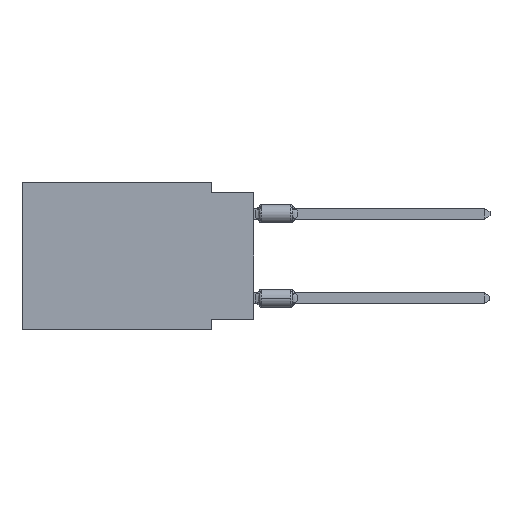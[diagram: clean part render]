
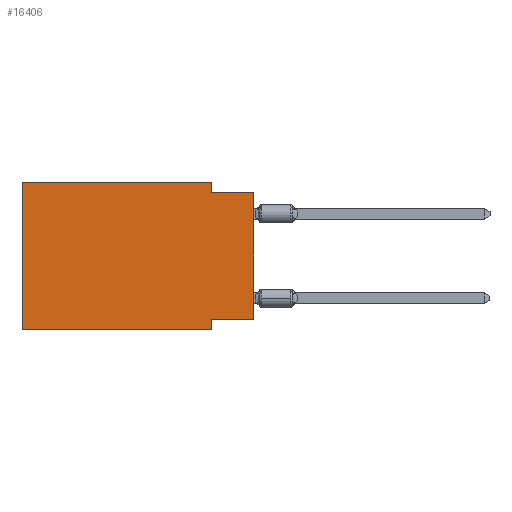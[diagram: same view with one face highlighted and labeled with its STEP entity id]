
A CAD part, left-side view. The second image highlights one B-rep face of the part: STEP entity #16406.
In plain terms, the highlighted planar face has unit normal (-1, 0, 0).
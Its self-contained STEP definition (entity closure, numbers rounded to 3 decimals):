
#138 = VERTEX_POINT ( 'NONE', #2093 ) ;
#1207 = EDGE_CURVE ( 'NONE', #15112, #24728, #23147, .T. ) ;
#1878 = VECTOR ( 'NONE', #22965, 1000. ) ;
#2093 = CARTESIAN_POINT ( 'NONE',  ( 0., 2.54, -0.635 ) ) ;
#2950 = VERTEX_POINT ( 'NONE', #10693 ) ;
#3107 = EDGE_CURVE ( 'NONE', #19279, #3376, #9127, .T. ) ;
#3235 = LINE ( 'NONE', #11205, #13302 ) ;
#3376 = VERTEX_POINT ( 'NONE', #8677 ) ;
#5197 = DIRECTION ( 'NONE',  ( 0., 0., 1. ) ) ;
#5227 = CARTESIAN_POINT ( 'NONE',  ( 0., 0., 0. ) ) ;
#5543 = PLANE ( 'NONE',  #12803 ) ;
#5921 = DIRECTION ( 'NONE',  ( 0., 0., -1. ) ) ;
#6563 = VECTOR ( 'NONE', #20011, 1000. ) ;
#6935 = VECTOR ( 'NONE', #16885, 1000. ) ;
#7129 = CARTESIAN_POINT ( 'NONE',  ( 0., 0., -8.255 ) ) ;
#7851 = LINE ( 'NONE', #25248, #24149 ) ;
#8677 = CARTESIAN_POINT ( 'NONE',  ( 0., 13.97, 0. ) ) ;
#9127 = LINE ( 'NONE', #9378, #20987 ) ;
#9378 = CARTESIAN_POINT ( 'NONE',  ( 0., 13.97, 0. ) ) ;
#9499 = EDGE_CURVE ( 'NONE', #2950, #11166, #7851, .T. ) ;
#10050 = CARTESIAN_POINT ( 'NONE',  ( 0., 2.54, -8.89 ) ) ;
#10204 = EDGE_CURVE ( 'NONE', #138, #24728, #3235, .T. ) ;
#10693 = CARTESIAN_POINT ( 'NONE',  ( 0., 2.54, -8.255 ) ) ;
#10913 = CARTESIAN_POINT ( 'NONE',  ( 0., 0., -8.255 ) ) ;
#11166 = VERTEX_POINT ( 'NONE', #10050 ) ;
#11205 = CARTESIAN_POINT ( 'NONE',  ( 0., 0., -0.635 ) ) ;
#11546 = DIRECTION ( 'NONE',  ( 1., 0., 0. ) ) ;
#11623 = VERTEX_POINT ( 'NONE', #20486 ) ;
#12564 = VECTOR ( 'NONE', #25693, 1000. ) ;
#12581 = ORIENTED_EDGE ( 'NONE', *, *, #13515, .F. ) ;
#12803 = AXIS2_PLACEMENT_3D ( 'NONE', #13507, #11546, #5921 ) ;
#13296 = CARTESIAN_POINT ( 'NONE',  ( 0., 13.97, -8.89 ) ) ;
#13302 = VECTOR ( 'NONE', #17094, 1000. ) ;
#13507 = CARTESIAN_POINT ( 'NONE',  ( 0., 13.97, 0. ) ) ;
#13515 = EDGE_CURVE ( 'NONE', #11623, #138, #17726, .T. ) ;
#13954 = VECTOR ( 'NONE', #16848, 1000. ) ;
#14031 = ORIENTED_EDGE ( 'NONE', *, *, #17161, .F. ) ;
#14717 = LINE ( 'NONE', #7129, #1878 ) ;
#15112 = VERTEX_POINT ( 'NONE', #10913 ) ;
#15865 = FACE_OUTER_BOUND ( 'NONE', #17742, .T. ) ;
#16216 = CARTESIAN_POINT ( 'NONE',  ( 0., 13.97, 0. ) ) ;
#16275 = ORIENTED_EDGE ( 'NONE', *, *, #3107, .F. ) ;
#16406 = ADVANCED_FACE ( 'NONE', ( #15865 ), #5543, .F. ) ;
#16848 = DIRECTION ( 'NONE',  ( 0., -1., 0. ) ) ;
#16885 = DIRECTION ( 'NONE',  ( 0., 0., 1. ) ) ;
#17094 = DIRECTION ( 'NONE',  ( 0., -1., 0. ) ) ;
#17161 = EDGE_CURVE ( 'NONE', #3376, #11623, #18188, .T. ) ;
#17664 = DIRECTION ( 'NONE',  ( 0., 0., -1. ) ) ;
#17668 = CARTESIAN_POINT ( 'NONE',  ( 0., 0., -0.635 ) ) ;
#17726 = LINE ( 'NONE', #21649, #12564 ) ;
#17742 = EDGE_LOOP ( 'NONE', ( #23379, #25678, #12581, #14031, #16275, #23564, #17910, #25296 ) ) ;
#17910 = ORIENTED_EDGE ( 'NONE', *, *, #9499, .F. ) ;
#18188 = LINE ( 'NONE', #16216, #6563 ) ;
#19279 = VERTEX_POINT ( 'NONE', #22698 ) ;
#20011 = DIRECTION ( 'NONE',  ( 0., -1., 0. ) ) ;
#20113 = EDGE_CURVE ( 'NONE', #19279, #11166, #24694, .T. ) ;
#20486 = CARTESIAN_POINT ( 'NONE',  ( 0., 2.54, 0. ) ) ;
#20547 = EDGE_CURVE ( 'NONE', #15112, #2950, #14717, .T. ) ;
#20987 = VECTOR ( 'NONE', #5197, 1000. ) ;
#21649 = CARTESIAN_POINT ( 'NONE',  ( 0., 2.54, 0. ) ) ;
#22698 = CARTESIAN_POINT ( 'NONE',  ( 0., 13.97, -8.89 ) ) ;
#22965 = DIRECTION ( 'NONE',  ( 0., 1., 0. ) ) ;
#23147 = LINE ( 'NONE', #5227, #6935 ) ;
#23379 = ORIENTED_EDGE ( 'NONE', *, *, #1207, .T. ) ;
#23564 = ORIENTED_EDGE ( 'NONE', *, *, #20113, .T. ) ;
#24149 = VECTOR ( 'NONE', #17664, 1000. ) ;
#24694 = LINE ( 'NONE', #13296, #13954 ) ;
#24728 = VERTEX_POINT ( 'NONE', #17668 ) ;
#25248 = CARTESIAN_POINT ( 'NONE',  ( 0., 2.54, -8.89 ) ) ;
#25296 = ORIENTED_EDGE ( 'NONE', *, *, #20547, .F. ) ;
#25678 = ORIENTED_EDGE ( 'NONE', *, *, #10204, .F. ) ;
#25693 = DIRECTION ( 'NONE',  ( 0., 0., -1. ) ) ;
